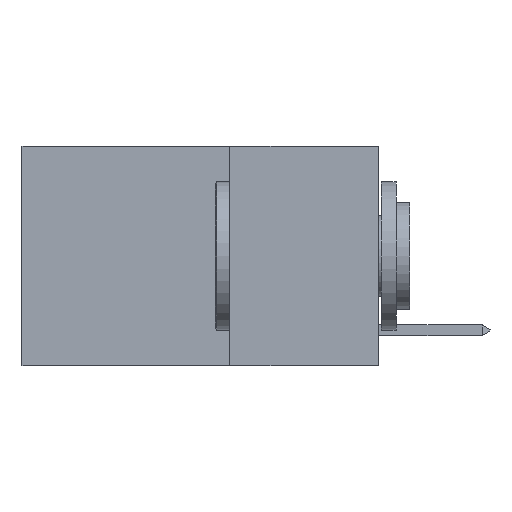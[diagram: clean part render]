
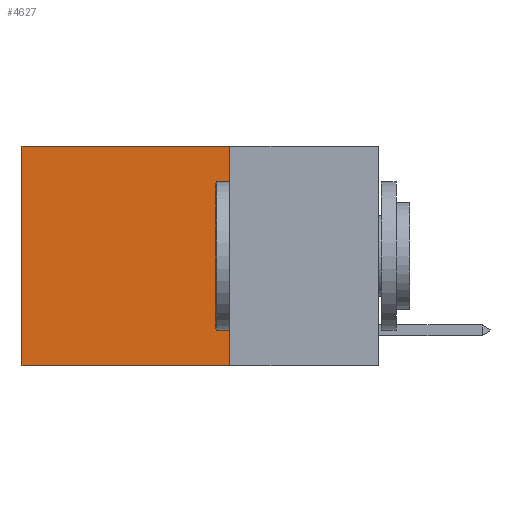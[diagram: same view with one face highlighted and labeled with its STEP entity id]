
A CAD part, left-side view. The second image highlights one B-rep face of the part: STEP entity #4627.
In plain terms, the highlighted planar face has unit normal (-1, 0, 0).
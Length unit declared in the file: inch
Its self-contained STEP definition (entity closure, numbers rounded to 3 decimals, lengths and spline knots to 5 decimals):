
#532 = EDGE_CURVE ( 'NONE', #18048, #15058, #4363, .T. ) ;
#630 = VECTOR ( 'NONE', #7937, 39.37008 ) ;
#1015 = VERTEX_POINT ( 'NONE', #7247 ) ;
#1642 = PLANE ( 'NONE',  #15581 ) ;
#2061 = CARTESIAN_POINT ( 'NONE',  ( 0.2625, 0.6, 0. ) ) ;
#2107 = ORIENTED_EDGE ( 'NONE', *, *, #532, .T. ) ;
#2611 = VECTOR ( 'NONE', #16166, 39.37008 ) ;
#3703 = CARTESIAN_POINT ( 'NONE',  ( 0.2625, 0.25, 0. ) ) ;
#4126 = LINE ( 'NONE', #3703, #2611 ) ;
#4363 = LINE ( 'NONE', #5169, #630 ) ;
#4627 = ADVANCED_FACE ( 'NONE', ( #11608 ), #1642, .F. ) ;
#5169 = CARTESIAN_POINT ( 'NONE',  ( 0.2625, 0.6, 0. ) ) ;
#5324 = EDGE_CURVE ( 'NONE', #8572, #1015, #9786, .T. ) ;
#5741 = VECTOR ( 'NONE', #7073, 39.37008 ) ;
#7012 = CARTESIAN_POINT ( 'NONE',  ( 0.2625, 0.25, -0.37 ) ) ;
#7073 = DIRECTION ( 'NONE',  ( 0., 1., 0. ) ) ;
#7219 = CARTESIAN_POINT ( 'NONE',  ( 0.2625, 0.25, 0. ) ) ;
#7247 = CARTESIAN_POINT ( 'NONE',  ( 0.2625, 0.25, -0.37 ) ) ;
#7937 = DIRECTION ( 'NONE',  ( 0., 0., -1. ) ) ;
#7968 = CARTESIAN_POINT ( 'NONE',  ( 0.2625, 0.6, -0.37 ) ) ;
#8357 = EDGE_CURVE ( 'NONE', #8572, #18048, #4126, .T. ) ;
#8572 = VERTEX_POINT ( 'NONE', #16346 ) ;
#8671 = VECTOR ( 'NONE', #10648, 39.37008 ) ;
#9536 = LINE ( 'NONE', #7012, #5741 ) ;
#9786 = LINE ( 'NONE', #15985, #8671 ) ;
#10121 = ORIENTED_EDGE ( 'NONE', *, *, #5324, .F. ) ;
#10648 = DIRECTION ( 'NONE',  ( 0., 0., -1. ) ) ;
#11608 = FACE_OUTER_BOUND ( 'NONE', #17122, .T. ) ;
#13581 = ORIENTED_EDGE ( 'NONE', *, *, #15011, .F. ) ;
#14261 = DIRECTION ( 'NONE',  ( 0., 0., -1. ) ) ;
#15011 = EDGE_CURVE ( 'NONE', #1015, #15058, #9536, .T. ) ;
#15058 = VERTEX_POINT ( 'NONE', #7968 ) ;
#15581 = AXIS2_PLACEMENT_3D ( 'NONE', #7219, #15787, #14261 ) ;
#15787 = DIRECTION ( 'NONE',  ( 1., 0., 0. ) ) ;
#15985 = CARTESIAN_POINT ( 'NONE',  ( 0.2625, 0.25, 0. ) ) ;
#16166 = DIRECTION ( 'NONE',  ( 0., 1., 0. ) ) ;
#16346 = CARTESIAN_POINT ( 'NONE',  ( 0.2625, 0.25, 0. ) ) ;
#16728 = ORIENTED_EDGE ( 'NONE', *, *, #8357, .T. ) ;
#17122 = EDGE_LOOP ( 'NONE', ( #2107, #13581, #10121, #16728 ) ) ;
#18048 = VERTEX_POINT ( 'NONE', #2061 ) ;
